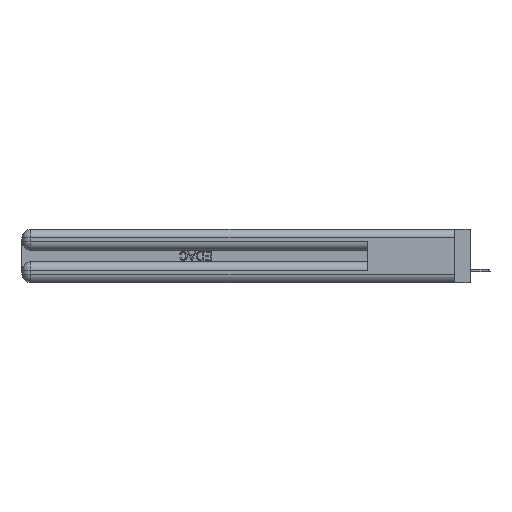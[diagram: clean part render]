
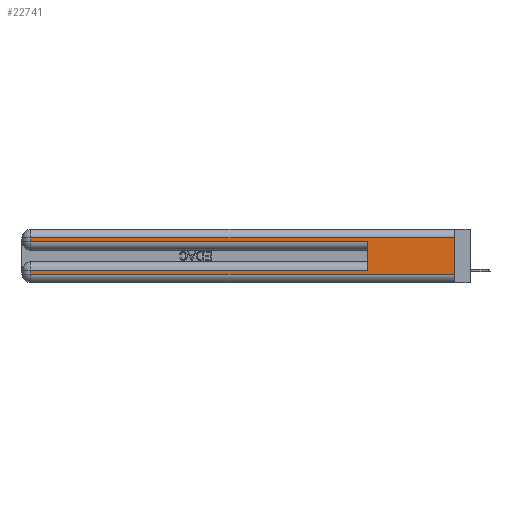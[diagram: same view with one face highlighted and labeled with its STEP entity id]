
A CAD part, left-side view. The second image highlights one B-rep face of the part: STEP entity #22741.
In plain terms, the highlighted planar face has unit normal (-1, 0, 0).
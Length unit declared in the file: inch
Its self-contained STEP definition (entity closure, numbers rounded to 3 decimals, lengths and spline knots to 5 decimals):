
#114 = VERTEX_POINT ( 'NONE', #1250 ) ;
#543 = EDGE_CURVE ( 'NONE', #931, #40378, #19171, .T. ) ;
#699 = ORIENTED_EDGE ( 'NONE', *, *, #20611, .F. ) ;
#931 = VERTEX_POINT ( 'NONE', #37604 ) ;
#1193 = LINE ( 'NONE', #46317, #31189 ) ;
#1250 = CARTESIAN_POINT ( 'NONE',  ( 0., 2.94, 0.31 ) ) ;
#4457 = VECTOR ( 'NONE', #26016, 39.37008 ) ;
#6660 = CARTESIAN_POINT ( 'NONE',  ( 0., 0., 0.285 ) ) ;
#7791 = EDGE_CURVE ( 'NONE', #13083, #33004, #21795, .T. ) ;
#8407 = VERTEX_POINT ( 'NONE', #38230 ) ;
#8472 = ORIENTED_EDGE ( 'NONE', *, *, #543, .T. ) ;
#9507 = CARTESIAN_POINT ( 'NONE',  ( 0., 2.94, 0.37 ) ) ;
#10246 = DIRECTION ( 'NONE',  ( 1., 0., 0. ) ) ;
#10809 = CARTESIAN_POINT ( 'NONE',  ( 0., 0., 0.31 ) ) ;
#11184 = ORIENTED_EDGE ( 'NONE', *, *, #7791, .F. ) ;
#13083 = VERTEX_POINT ( 'NONE', #10809 ) ;
#14543 = CARTESIAN_POINT ( 'NONE',  ( 0., 2.94, 0.285 ) ) ;
#15145 = PLANE ( 'NONE',  #38601 ) ;
#16698 = VECTOR ( 'NONE', #47965, 39.37008 ) ;
#17898 = CARTESIAN_POINT ( 'NONE',  ( 0., 0., 0.06 ) ) ;
#19171 = LINE ( 'NONE', #41863, #45973 ) ;
#20611 = EDGE_CURVE ( 'NONE', #47433, #8407, #46622, .T. ) ;
#21074 = LINE ( 'NONE', #9507, #33665 ) ;
#21138 = VECTOR ( 'NONE', #30588, 39.37008 ) ;
#21795 = LINE ( 'NONE', #22274, #16698 ) ;
#21796 = DIRECTION ( 'NONE',  ( 0., 0., -1. ) ) ;
#21918 = LINE ( 'NONE', #6660, #25193 ) ;
#22274 = CARTESIAN_POINT ( 'NONE',  ( 0., 0., 0.37 ) ) ;
#22741 = ADVANCED_FACE ( 'NONE', ( #29202 ), #15145, .F. ) ;
#23680 = CARTESIAN_POINT ( 'NONE',  ( 0., 0.6, 0.145 ) ) ;
#25193 = VECTOR ( 'NONE', #41153, 39.37008 ) ;
#25613 = ORIENTED_EDGE ( 'NONE', *, *, #28471, .T. ) ;
#25667 = ORIENTED_EDGE ( 'NONE', *, *, #32674, .T. ) ;
#25840 = LINE ( 'NONE', #30522, #35158 ) ;
#26016 = DIRECTION ( 'NONE',  ( 0., -1., 0. ) ) ;
#26518 = EDGE_CURVE ( 'NONE', #47433, #931, #1193, .T. ) ;
#26734 = EDGE_CURVE ( 'NONE', #40378, #33004, #43324, .T. ) ;
#28471 = EDGE_CURVE ( 'NONE', #114, #35509, #21074, .T. ) ;
#29202 = FACE_OUTER_BOUND ( 'NONE', #30779, .T. ) ;
#30169 = ORIENTED_EDGE ( 'NONE', *, *, #26518, .T. ) ;
#30522 = CARTESIAN_POINT ( 'NONE',  ( 0., 0., 0.31 ) ) ;
#30588 = DIRECTION ( 'NONE',  ( 0., 0., 1. ) ) ;
#30779 = EDGE_LOOP ( 'NONE', ( #11184, #30935, #25613, #25667, #699, #30169, #8472, #47032 ) ) ;
#30935 = ORIENTED_EDGE ( 'NONE', *, *, #47263, .T. ) ;
#31189 = VECTOR ( 'NONE', #46552, 39.37008 ) ;
#32674 = EDGE_CURVE ( 'NONE', #35509, #8407, #21918, .T. ) ;
#33004 = VERTEX_POINT ( 'NONE', #17898 ) ;
#33404 = CARTESIAN_POINT ( 'NONE',  ( 0., 0., 0.06 ) ) ;
#33621 = DIRECTION ( 'NONE',  ( 0., 0., -1. ) ) ;
#33665 = VECTOR ( 'NONE', #21796, 39.37008 ) ;
#34699 = DIRECTION ( 'NONE',  ( 0., 0., -1. ) ) ;
#35158 = VECTOR ( 'NONE', #45574, 39.37008 ) ;
#35509 = VERTEX_POINT ( 'NONE', #14543 ) ;
#36199 = CARTESIAN_POINT ( 'NONE',  ( 0., 2.94, 0.06 ) ) ;
#37604 = CARTESIAN_POINT ( 'NONE',  ( 0., 2.94, 0.085 ) ) ;
#38230 = CARTESIAN_POINT ( 'NONE',  ( 0., 0.6, 0.285 ) ) ;
#38601 = AXIS2_PLACEMENT_3D ( 'NONE', #40812, #10246, #33621 ) ;
#39382 = CARTESIAN_POINT ( 'NONE',  ( 0., 0.6, 0.085 ) ) ;
#40378 = VERTEX_POINT ( 'NONE', #36199 ) ;
#40812 = CARTESIAN_POINT ( 'NONE',  ( 0., 0., 0.37 ) ) ;
#41153 = DIRECTION ( 'NONE',  ( 0., -1., 0. ) ) ;
#41863 = CARTESIAN_POINT ( 'NONE',  ( 0., 2.94, 0.37 ) ) ;
#43324 = LINE ( 'NONE', #33404, #4457 ) ;
#45574 = DIRECTION ( 'NONE',  ( 0., 1., 0. ) ) ;
#45973 = VECTOR ( 'NONE', #34699, 39.37008 ) ;
#46317 = CARTESIAN_POINT ( 'NONE',  ( 0., 0., 0.085 ) ) ;
#46552 = DIRECTION ( 'NONE',  ( 0., 1., 0. ) ) ;
#46622 = LINE ( 'NONE', #23680, #21138 ) ;
#47032 = ORIENTED_EDGE ( 'NONE', *, *, #26734, .T. ) ;
#47263 = EDGE_CURVE ( 'NONE', #13083, #114, #25840, .T. ) ;
#47433 = VERTEX_POINT ( 'NONE', #39382 ) ;
#47965 = DIRECTION ( 'NONE',  ( 0., 0., -1. ) ) ;
